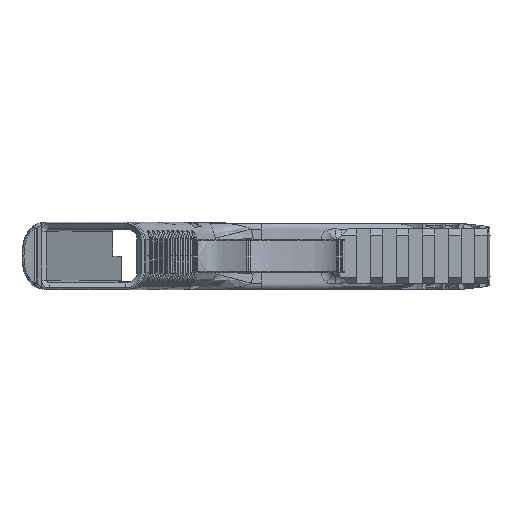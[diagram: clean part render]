
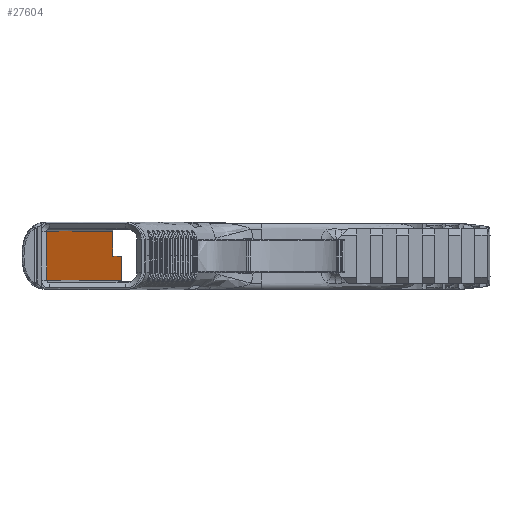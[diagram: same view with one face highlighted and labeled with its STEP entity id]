
A CAD part, top view. The second image highlights one B-rep face of the part: STEP entity #27604.
In plain terms, the highlighted planar face has unit normal (0.951, 0, 0.309).
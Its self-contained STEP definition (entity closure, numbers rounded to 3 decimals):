
#384 = DIRECTION ( 'NONE',  ( -0.951, 0., -0.309 ) ) ;
#1535 = VERTEX_POINT ( 'NONE', #17609 ) ;
#1599 = LINE ( 'NONE', #20299, #49729 ) ;
#6055 = VECTOR ( 'NONE', #47398, 1000. ) ;
#8351 = CARTESIAN_POINT ( 'NONE',  ( 24.128, -9.399, -10.543 ) ) ;
#11050 = VECTOR ( 'NONE', #54171, 1000. ) ;
#11148 = EDGE_CURVE ( 'NONE', #67500, #42721, #36229, .T. ) ;
#11398 = AXIS2_PLACEMENT_3D ( 'NONE', #12644, #384, #63957 ) ;
#12644 = CARTESIAN_POINT ( 'NONE',  ( 52.695, 0., -98.462 ) ) ;
#15085 = DIRECTION ( 'NONE',  ( 0.309, 0., -0.951 ) ) ;
#16448 = ORIENTED_EDGE ( 'NONE', *, *, #66294, .F. ) ;
#17609 = CARTESIAN_POINT ( 'NONE',  ( 49.444, 9.399, -88.458 ) ) ;
#20299 = CARTESIAN_POINT ( 'NONE',  ( 52.695, 9.399, -98.462 ) ) ;
#22197 = CARTESIAN_POINT ( 'NONE',  ( 52.695, 0.002, -98.462 ) ) ;
#22456 = DIRECTION ( 'NONE',  ( 0., 1., 0. ) ) ;
#24050 = CARTESIAN_POINT ( 'NONE',  ( 52.856, 0.001, -98.958 ) ) ;
#25374 = CARTESIAN_POINT ( 'NONE',  ( 52.856, -9.399, -98.958 ) ) ;
#25475 = EDGE_CURVE ( 'NONE', #50925, #30551, #56038, .T. ) ;
#27604 = ADVANCED_FACE ( 'NONE', ( #73187 ), #28762, .F. ) ;
#27628 = CARTESIAN_POINT ( 'NONE',  ( 49.444, 0.002, -88.458 ) ) ;
#28762 = PLANE ( 'NONE',  #11398 ) ;
#28924 = VERTEX_POINT ( 'NONE', #25374 ) ;
#30551 = VERTEX_POINT ( 'NONE', #33188 ) ;
#32878 = LINE ( 'NONE', #42321, #46237 ) ;
#32905 = EDGE_CURVE ( 'NONE', #30551, #28924, #73879, .T. ) ;
#33141 = EDGE_CURVE ( 'NONE', #42721, #1535, #1599, .T. ) ;
#33188 = CARTESIAN_POINT ( 'NONE',  ( 52.856, 0.002, -98.958 ) ) ;
#35494 = EDGE_LOOP ( 'NONE', ( #16448, #63894, #66038, #37322, #58624, #42226 ) ) ;
#36229 = LINE ( 'NONE', #67622, #39808 ) ;
#37322 = ORIENTED_EDGE ( 'NONE', *, *, #58159, .F. ) ;
#39808 = VECTOR ( 'NONE', #22456, 1000. ) ;
#41692 = VECTOR ( 'NONE', #44573, 1000. ) ;
#42226 = ORIENTED_EDGE ( 'NONE', *, *, #25475, .F. ) ;
#42321 = CARTESIAN_POINT ( 'NONE',  ( 49.444, 0., -88.458 ) ) ;
#42721 = VERTEX_POINT ( 'NONE', #46551 ) ;
#44573 = DIRECTION ( 'NONE',  ( 0.309, 0., -0.951 ) ) ;
#46237 = VECTOR ( 'NONE', #47570, 1000. ) ;
#46551 = CARTESIAN_POINT ( 'NONE',  ( 24.128, 9.399, -10.543 ) ) ;
#47398 = DIRECTION ( 'NONE',  ( 0., -1., 0. ) ) ;
#47570 = DIRECTION ( 'NONE',  ( 0., -1., 0. ) ) ;
#49729 = VECTOR ( 'NONE', #15085, 1000. ) ;
#50925 = VERTEX_POINT ( 'NONE', #27628 ) ;
#53437 = CARTESIAN_POINT ( 'NONE',  ( 52.695, -9.399, -98.462 ) ) ;
#54171 = DIRECTION ( 'NONE',  ( -0.309, 0., 0.951 ) ) ;
#56038 = LINE ( 'NONE', #22197, #41692 ) ;
#58159 = EDGE_CURVE ( 'NONE', #28924, #67500, #73502, .T. ) ;
#58624 = ORIENTED_EDGE ( 'NONE', *, *, #32905, .F. ) ;
#63894 = ORIENTED_EDGE ( 'NONE', *, *, #33141, .F. ) ;
#63957 = DIRECTION ( 'NONE',  ( -0.309, 0., 0.951 ) ) ;
#66038 = ORIENTED_EDGE ( 'NONE', *, *, #11148, .F. ) ;
#66294 = EDGE_CURVE ( 'NONE', #1535, #50925, #32878, .T. ) ;
#67500 = VERTEX_POINT ( 'NONE', #8351 ) ;
#67622 = CARTESIAN_POINT ( 'NONE',  ( 24.128, 0., -10.543 ) ) ;
#73187 = FACE_OUTER_BOUND ( 'NONE', #35494, .T. ) ;
#73502 = LINE ( 'NONE', #53437, #11050 ) ;
#73879 = LINE ( 'NONE', #24050, #6055 ) ;
